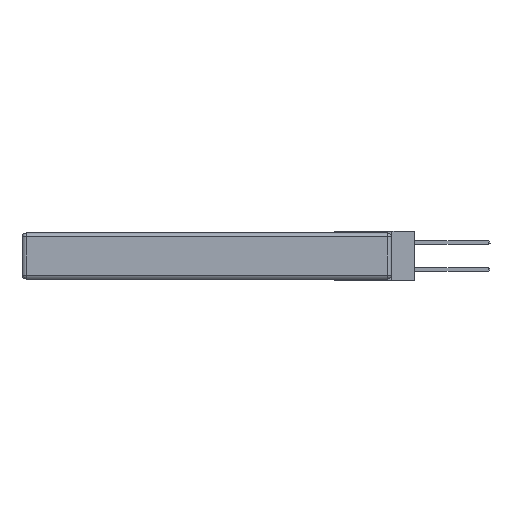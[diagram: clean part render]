
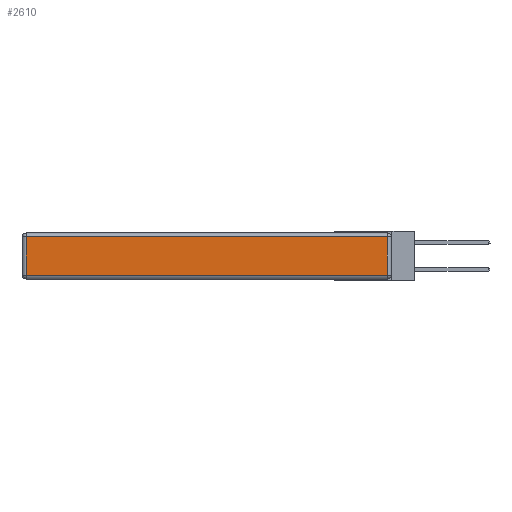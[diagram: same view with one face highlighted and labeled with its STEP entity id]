
A CAD part, left-side view. The second image highlights one B-rep face of the part: STEP entity #2610.
In plain terms, the highlighted planar face has unit normal (-1, 0, 0).
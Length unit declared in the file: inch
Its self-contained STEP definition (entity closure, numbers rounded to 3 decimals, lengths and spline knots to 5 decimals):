
#1624 = ORIENTED_EDGE ( 'NONE', *, *, #21357, .T. ) ;
#2610 = ADVANCED_FACE ( 'NONE', ( #30358 ), #31859, .T. ) ;
#2946 = VECTOR ( 'NONE', #21115, 39.37008 ) ;
#4210 = LINE ( 'NONE', #23727, #11807 ) ;
#4212 = CARTESIAN_POINT ( 'NONE',  ( 0., 2.72, -0.343 ) ) ;
#6293 = DIRECTION ( 'NONE',  ( 0., -1., 0. ) ) ;
#6736 = DIRECTION ( 'NONE',  ( 0., 0., -1. ) ) ;
#6869 = ORIENTED_EDGE ( 'NONE', *, *, #28428, .T. ) ;
#7391 = CARTESIAN_POINT ( 'NONE',  ( 0., 2.72, -0.03 ) ) ;
#8681 = VECTOR ( 'NONE', #6736, 39.37008 ) ;
#9708 = LINE ( 'NONE', #28422, #2946 ) ;
#11066 = CARTESIAN_POINT ( 'NONE',  ( 0., 0.03, -0.03 ) ) ;
#11485 = LINE ( 'NONE', #4212, #8681 ) ;
#11807 = VECTOR ( 'NONE', #6293, 39.37008 ) ;
#12100 = VERTEX_POINT ( 'NONE', #15330 ) ;
#12332 = CARTESIAN_POINT ( 'NONE',  ( 0., 2.75, -0.03 ) ) ;
#12550 = DIRECTION ( 'NONE',  ( 0., 1., 0. ) ) ;
#13579 = EDGE_CURVE ( 'NONE', #12100, #22353, #4210, .T. ) ;
#14273 = EDGE_LOOP ( 'NONE', ( #25367, #6869, #1624, #25613 ) ) ;
#15103 = VECTOR ( 'NONE', #12550, 39.37008 ) ;
#15330 = CARTESIAN_POINT ( 'NONE',  ( 0., 2.72, -0.313 ) ) ;
#15626 = VERTEX_POINT ( 'NONE', #11066 ) ;
#16694 = DIRECTION ( 'NONE',  ( 0., 0., 1. ) ) ;
#18936 = AXIS2_PLACEMENT_3D ( 'NONE', #24007, #29413, #16694 ) ;
#21115 = DIRECTION ( 'NONE',  ( 0., 0., 1. ) ) ;
#21357 = EDGE_CURVE ( 'NONE', #15626, #27944, #30126, .T. ) ;
#22353 = VERTEX_POINT ( 'NONE', #29478 ) ;
#23727 = CARTESIAN_POINT ( 'NONE',  ( 0., 0., -0.313 ) ) ;
#24007 = CARTESIAN_POINT ( 'NONE',  ( 0., 0., -0.343 ) ) ;
#25367 = ORIENTED_EDGE ( 'NONE', *, *, #13579, .T. ) ;
#25613 = ORIENTED_EDGE ( 'NONE', *, *, #30914, .T. ) ;
#27944 = VERTEX_POINT ( 'NONE', #7391 ) ;
#28422 = CARTESIAN_POINT ( 'NONE',  ( 0., 0.03, -0.343 ) ) ;
#28428 = EDGE_CURVE ( 'NONE', #22353, #15626, #9708, .T. ) ;
#29413 = DIRECTION ( 'NONE',  ( -1., 0., 0. ) ) ;
#29478 = CARTESIAN_POINT ( 'NONE',  ( 0., 0.03, -0.313 ) ) ;
#30126 = LINE ( 'NONE', #12332, #15103 ) ;
#30358 = FACE_OUTER_BOUND ( 'NONE', #14273, .T. ) ;
#30914 = EDGE_CURVE ( 'NONE', #27944, #12100, #11485, .T. ) ;
#31859 = PLANE ( 'NONE',  #18936 ) ;
